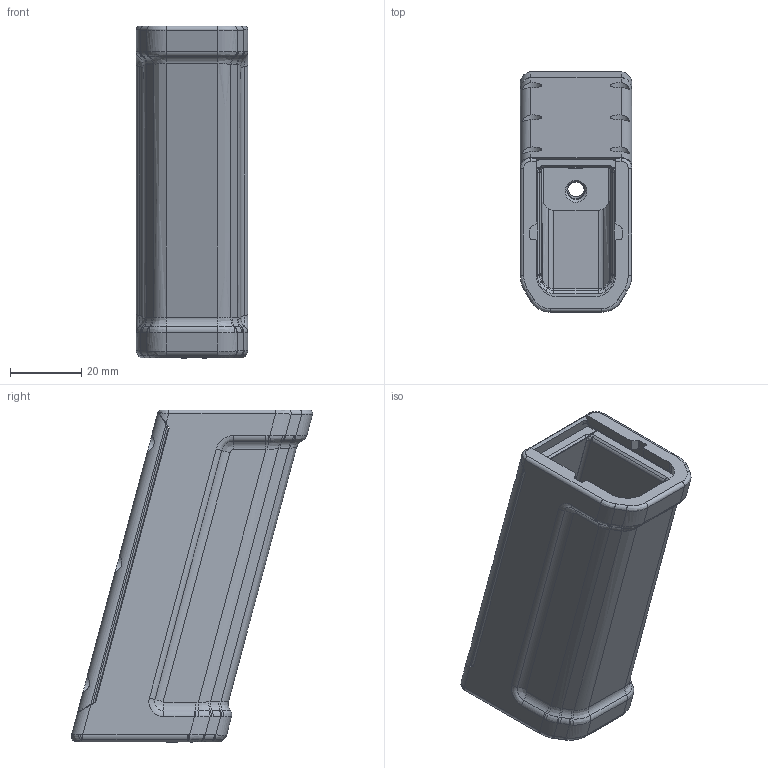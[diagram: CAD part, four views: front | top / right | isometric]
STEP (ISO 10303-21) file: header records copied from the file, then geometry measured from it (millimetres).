
FILE_DESCRIPTION(/* description */ (''),/* implementation_level */ '2;1');
FILE_NAME(/* name */ 'Final Concept.step',/* time_stamp */ '2021-08-16T05:15:40-04:00',/* author */ (''),/* organization */ (''),/* preprocessor_version */ 'ST-DEVELOPER v18.1',/* originating_system */ 'Autodesk Translation Framework v10.9.0.1377',/* authorisation */ '');
FILE_SCHEMA (('AUTOMOTIVE_DESIGN { 1 0 10303 214 3 1 1 }'));
Length unit declared in the file: millimetre
Products named in the file (1): Final Concept
Bounding box: 31.28 x 67.63 x 93.14 mm (x, y, z)
Volume: 50913.6 mm3; surface area: 27873 mm2
Topology: 2 solids, 2 shells, 375 faces, 930 edges, 570 vertices
Faces by surface type: bspline 161, cylinder 119, plane 85, cone 6, torus 4
Full cylindrical faces by diameter (mm): 2.8 x12, 5.5 x6, 14.521 x1, 16.771 x1
Entity records: 14127 total; most frequent: CARTESIAN_POINT 5928, ORIENTED_EDGE 1860, DIRECTION 1430, EDGE_CURVE 930, VERTEX_POINT 570, AXIS2_PLACEMENT_3D 544, EDGE_LOOP 400, FACE_OUTER_BOUND 375
